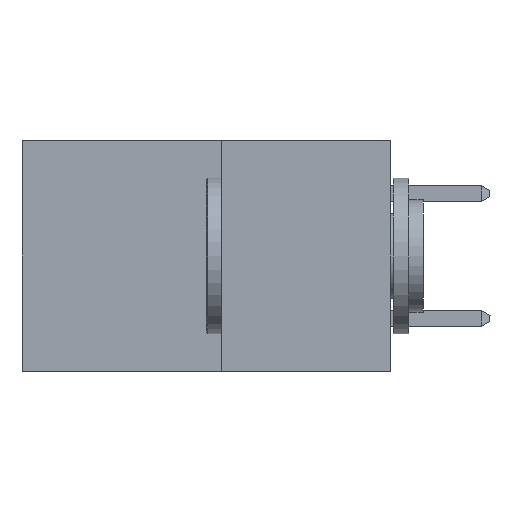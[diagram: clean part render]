
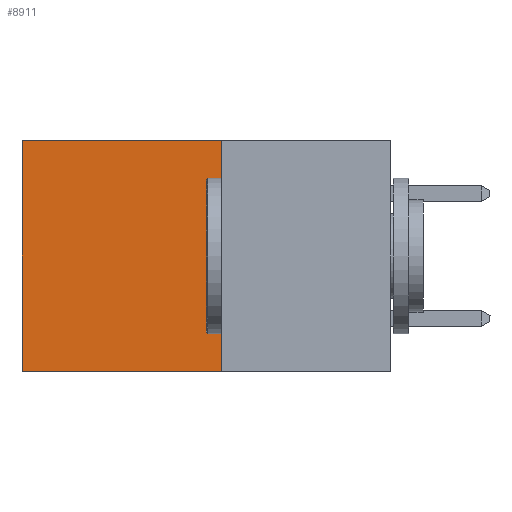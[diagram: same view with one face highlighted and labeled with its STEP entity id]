
A CAD part, left-side view. The second image highlights one B-rep face of the part: STEP entity #8911.
In plain terms, the highlighted planar face has unit normal (-1, 0, 0).
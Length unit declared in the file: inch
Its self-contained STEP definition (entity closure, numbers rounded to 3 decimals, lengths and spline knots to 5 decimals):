
#94 = DIRECTION ( 'NONE',  ( 0., 0., -1. ) ) ;
#144 = ORIENTED_EDGE ( 'NONE', *, *, #731, .T. ) ;
#345 = LINE ( 'NONE', #5935, #8352 ) ;
#731 = EDGE_CURVE ( 'NONE', #6576, #4557, #345, .T. ) ;
#1003 = CARTESIAN_POINT ( 'NONE',  ( 0.277, 0.27, -0.37 ) ) ;
#1304 = CARTESIAN_POINT ( 'NONE',  ( 0.277, 0.27, 0. ) ) ;
#1711 = DIRECTION ( 'NONE',  ( 0., 1., 0. ) ) ;
#1763 = CARTESIAN_POINT ( 'NONE',  ( 0.277, 0.27, -0.37 ) ) ;
#4293 = ORIENTED_EDGE ( 'NONE', *, *, #5656, .F. ) ;
#4379 = VECTOR ( 'NONE', #5147, 39.37008 ) ;
#4416 = VECTOR ( 'NONE', #1711, 39.37008 ) ;
#4557 = VERTEX_POINT ( 'NONE', #8693 ) ;
#4984 = DIRECTION ( 'NONE',  ( 1., 0., 0. ) ) ;
#5147 = DIRECTION ( 'NONE',  ( 0., 0., -1. ) ) ;
#5164 = FACE_OUTER_BOUND ( 'NONE', #7304, .T. ) ;
#5656 = EDGE_CURVE ( 'NONE', #5806, #6049, #6397, .T. ) ;
#5806 = VERTEX_POINT ( 'NONE', #1003 ) ;
#5866 = DIRECTION ( 'NONE',  ( 0., 0., -1. ) ) ;
#5900 = CARTESIAN_POINT ( 'NONE',  ( 0.277, 0.59, -0.37 ) ) ;
#5935 = CARTESIAN_POINT ( 'NONE',  ( 0.277, 0.27, 0. ) ) ;
#6049 = VERTEX_POINT ( 'NONE', #6358 ) ;
#6280 = ORIENTED_EDGE ( 'NONE', *, *, #8323, .F. ) ;
#6355 = LINE ( 'NONE', #8045, #4379 ) ;
#6358 = CARTESIAN_POINT ( 'NONE',  ( 0.277, 0.59, -0.37 ) ) ;
#6368 = EDGE_CURVE ( 'NONE', #4557, #6049, #7163, .T. ) ;
#6397 = LINE ( 'NONE', #1763, #4416 ) ;
#6576 = VERTEX_POINT ( 'NONE', #1304 ) ;
#6950 = VECTOR ( 'NONE', #5866, 39.37008 ) ;
#7163 = LINE ( 'NONE', #5900, #6950 ) ;
#7304 = EDGE_LOOP ( 'NONE', ( #9881, #4293, #6280, #144 ) ) ;
#7879 = PLANE ( 'NONE',  #8163 ) ;
#8045 = CARTESIAN_POINT ( 'NONE',  ( 0.277, 0.27, -0.37 ) ) ;
#8163 = AXIS2_PLACEMENT_3D ( 'NONE', #9350, #4984, #94 ) ;
#8323 = EDGE_CURVE ( 'NONE', #6576, #5806, #6355, .T. ) ;
#8352 = VECTOR ( 'NONE', #8576, 39.37008 ) ;
#8576 = DIRECTION ( 'NONE',  ( 0., 1., 0. ) ) ;
#8693 = CARTESIAN_POINT ( 'NONE',  ( 0.277, 0.59, 0. ) ) ;
#8911 = ADVANCED_FACE ( 'NONE', ( #5164 ), #7879, .F. ) ;
#9350 = CARTESIAN_POINT ( 'NONE',  ( 0.277, 0.27, -0.37 ) ) ;
#9881 = ORIENTED_EDGE ( 'NONE', *, *, #6368, .T. ) ;
